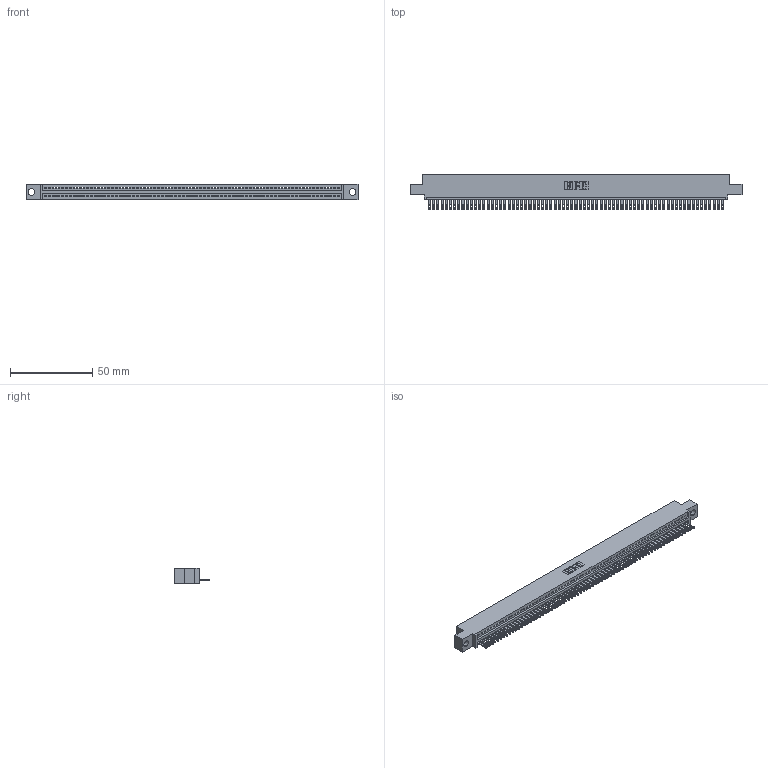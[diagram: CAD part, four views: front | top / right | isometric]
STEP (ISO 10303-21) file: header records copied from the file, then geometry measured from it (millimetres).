
FILE_DESCRIPTION (( 'STEP AP203' ), '1' );
FILE_NAME ('345-071-500-404.STEP', '2021-05-28T16:24:45', ( '' ), ( '' ), 'SwSTEP 2.0', 'SolidWorks 2020', '' );
FILE_SCHEMA (( 'CONFIG_CONTROL_DESIGN' ));
Length unit declared in the file: inch
Products named in the file (3): 345 Part_0.110 Offset - 0.156 Dia-TI; 345-292-001_345-293-100; 345-071-500-404
Assembly tree (72 placements, depth 2):
  345-071-500-404
    345 Part_0.110 Offset - 0.156 Dia-TI
    345-292-001_345-293-100  x71
Bounding box: 201.55 x 21.51 x 9.4 mm (x, y, z)
Volume: 19245.5 mm3; surface area: 26053.5 mm2
Topology: 72 solids, 72 shells, 3978 faces, 12317 edges, 8210 vertices
Faces by surface type: plane 2512, cylinder 1466
Entity records: 50013 total; most frequent: ORIENTED_EDGE 8674, CARTESIAN_POINT 8671, DIRECTION 7531, EDGE_CURVE 4337, LINE 3917, VECTOR 3917, VERTEX_POINT 2890, AXIS2_PLACEMENT_3D 1807
